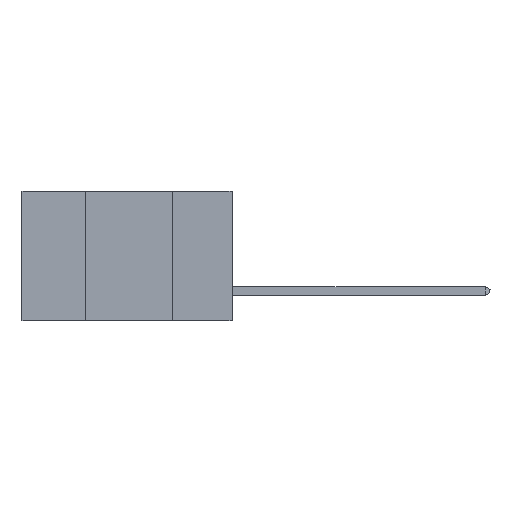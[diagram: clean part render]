
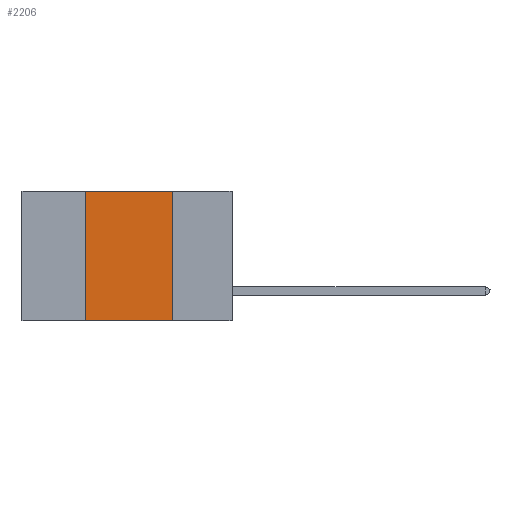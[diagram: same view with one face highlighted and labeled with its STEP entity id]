
A CAD part, left-side view. The second image highlights one B-rep face of the part: STEP entity #2206.
In plain terms, the highlighted planar face has unit normal (-1, 0, 0).
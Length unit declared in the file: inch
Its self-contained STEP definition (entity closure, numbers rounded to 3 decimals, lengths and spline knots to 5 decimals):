
#1026 = DIRECTION ( 'NONE',  ( 1., 0., 0. ) ) ;
#2206 = ADVANCED_FACE ( 'NONE', ( #7016 ), #11585, .F. ) ;
#2577 = VERTEX_POINT ( 'NONE', #6200 ) ;
#3566 = ORIENTED_EDGE ( 'NONE', *, *, #20583, .F. ) ;
#4392 = VECTOR ( 'NONE', #26574, 39.37008 ) ;
#6200 = CARTESIAN_POINT ( 'NONE',  ( 0., 0.42, -0.37 ) ) ;
#6903 = CARTESIAN_POINT ( 'NONE',  ( 0., 0.17, 0. ) ) ;
#7008 = LINE ( 'NONE', #28184, #34357 ) ;
#7016 = FACE_OUTER_BOUND ( 'NONE', #29484, .T. ) ;
#10848 = DIRECTION ( 'NONE',  ( 0., 0., 1. ) ) ;
#11434 = CARTESIAN_POINT ( 'NONE',  ( 0., 0.6, 0. ) ) ;
#11446 = CARTESIAN_POINT ( 'NONE',  ( 0., 0.42, 0. ) ) ;
#11585 = PLANE ( 'NONE',  #18828 ) ;
#13656 = LINE ( 'NONE', #35879, #21539 ) ;
#14409 = VERTEX_POINT ( 'NONE', #6903 ) ;
#15865 = VERTEX_POINT ( 'NONE', #44058 ) ;
#17322 = EDGE_CURVE ( 'NONE', #2577, #15865, #17919, .T. ) ;
#17919 = LINE ( 'NONE', #11446, #23619 ) ;
#18023 = DIRECTION ( 'NONE',  ( 0., 0., -1. ) ) ;
#18828 = AXIS2_PLACEMENT_3D ( 'NONE', #11434, #1026, #36119 ) ;
#20583 = EDGE_CURVE ( 'NONE', #15865, #14409, #42347, .T. ) ;
#20845 = CARTESIAN_POINT ( 'NONE',  ( 0., 0.17, -0.37 ) ) ;
#21539 = VECTOR ( 'NONE', #18023, 39.37008 ) ;
#23619 = VECTOR ( 'NONE', #10848, 39.37008 ) ;
#23652 = ORIENTED_EDGE ( 'NONE', *, *, #24477, .T. ) ;
#24477 = EDGE_CURVE ( 'NONE', #2577, #30352, #7008, .T. ) ;
#24915 = DIRECTION ( 'NONE',  ( 0., -1., 0. ) ) ;
#26574 = DIRECTION ( 'NONE',  ( 0., -1., 0. ) ) ;
#28184 = CARTESIAN_POINT ( 'NONE',  ( 0., 0.6, -0.37 ) ) ;
#29484 = EDGE_LOOP ( 'NONE', ( #32136, #3566, #40739, #23652 ) ) ;
#30352 = VERTEX_POINT ( 'NONE', #20845 ) ;
#32136 = ORIENTED_EDGE ( 'NONE', *, *, #46187, .F. ) ;
#34357 = VECTOR ( 'NONE', #24915, 39.37008 ) ;
#35879 = CARTESIAN_POINT ( 'NONE',  ( 0., 0.17, 0. ) ) ;
#36119 = DIRECTION ( 'NONE',  ( 0., 0., -1. ) ) ;
#37177 = CARTESIAN_POINT ( 'NONE',  ( 0., 0.6, 0. ) ) ;
#40739 = ORIENTED_EDGE ( 'NONE', *, *, #17322, .F. ) ;
#42347 = LINE ( 'NONE', #37177, #4392 ) ;
#44058 = CARTESIAN_POINT ( 'NONE',  ( 0., 0.42, 0. ) ) ;
#46187 = EDGE_CURVE ( 'NONE', #14409, #30352, #13656, .T. ) ;
